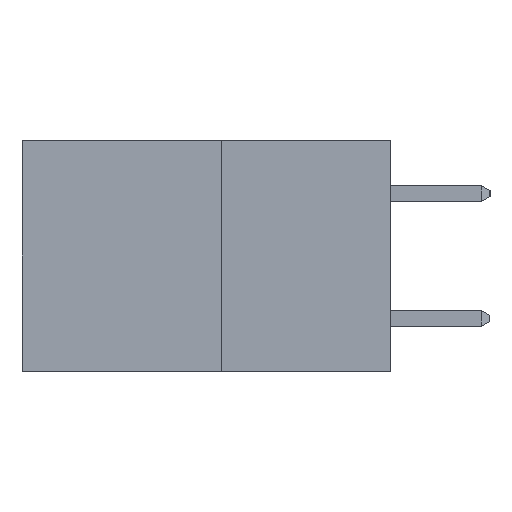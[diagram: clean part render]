
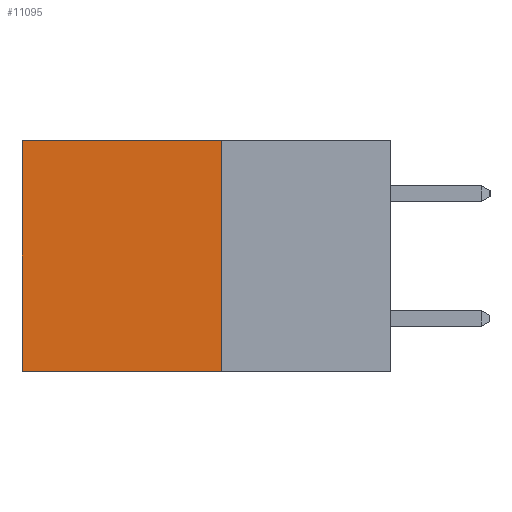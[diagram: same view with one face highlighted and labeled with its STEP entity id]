
A CAD part, left-side view. The second image highlights one B-rep face of the part: STEP entity #11095.
In plain terms, the highlighted planar face has unit normal (-1, 0, 0).
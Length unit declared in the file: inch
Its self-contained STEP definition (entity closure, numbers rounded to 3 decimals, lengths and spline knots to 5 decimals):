
#29 = LINE ( 'NONE', #15586, #6264 ) ;
#451 = ORIENTED_EDGE ( 'NONE', *, *, #4516, .T. ) ;
#937 = CARTESIAN_POINT ( 'NONE',  ( 0.277, 0.59, 0. ) ) ;
#2803 = EDGE_CURVE ( 'NONE', #3641, #4200, #3269, .T. ) ;
#3064 = DIRECTION ( 'NONE',  ( 1., 0., 0. ) ) ;
#3269 = LINE ( 'NONE', #3880, #9485 ) ;
#3363 = ORIENTED_EDGE ( 'NONE', *, *, #2803, .F. ) ;
#3641 = VERTEX_POINT ( 'NONE', #14148 ) ;
#3850 = VERTEX_POINT ( 'NONE', #6084 ) ;
#3880 = CARTESIAN_POINT ( 'NONE',  ( 0.277, 0.27, -0.37 ) ) ;
#4200 = VERTEX_POINT ( 'NONE', #7106 ) ;
#4208 = FACE_OUTER_BOUND ( 'NONE', #8446, .T. ) ;
#4516 = EDGE_CURVE ( 'NONE', #3641, #12582, #9625, .T. ) ;
#5011 = EDGE_CURVE ( 'NONE', #4200, #3850, #8862, .T. ) ;
#5184 = VECTOR ( 'NONE', #14505, 39.37008 ) ;
#5281 = DIRECTION ( 'NONE',  ( 0., 0., -1. ) ) ;
#5482 = AXIS2_PLACEMENT_3D ( 'NONE', #10503, #3064, #11690 ) ;
#5937 = ORIENTED_EDGE ( 'NONE', *, *, #7712, .T. ) ;
#6084 = CARTESIAN_POINT ( 'NONE',  ( 0.277, 0.59, -0.37 ) ) ;
#6264 = VECTOR ( 'NONE', #15557, 39.37008 ) ;
#7106 = CARTESIAN_POINT ( 'NONE',  ( 0.277, 0.27, -0.37 ) ) ;
#7712 = EDGE_CURVE ( 'NONE', #12582, #3850, #29, .T. ) ;
#8039 = PLANE ( 'NONE',  #5482 ) ;
#8446 = EDGE_LOOP ( 'NONE', ( #5937, #15397, #3363, #451 ) ) ;
#8862 = LINE ( 'NONE', #14587, #5184 ) ;
#9485 = VECTOR ( 'NONE', #5281, 39.37008 ) ;
#9625 = LINE ( 'NONE', #11759, #12398 ) ;
#10503 = CARTESIAN_POINT ( 'NONE',  ( 0.277, 0.27, -0.37 ) ) ;
#11095 = ADVANCED_FACE ( 'NONE', ( #4208 ), #8039, .F. ) ;
#11690 = DIRECTION ( 'NONE',  ( 0., 0., -1. ) ) ;
#11759 = CARTESIAN_POINT ( 'NONE',  ( 0.277, 0.27, 0. ) ) ;
#11859 = DIRECTION ( 'NONE',  ( 0., 1., 0. ) ) ;
#12398 = VECTOR ( 'NONE', #11859, 39.37008 ) ;
#12582 = VERTEX_POINT ( 'NONE', #937 ) ;
#14148 = CARTESIAN_POINT ( 'NONE',  ( 0.277, 0.27, 0. ) ) ;
#14505 = DIRECTION ( 'NONE',  ( 0., 1., 0. ) ) ;
#14587 = CARTESIAN_POINT ( 'NONE',  ( 0.277, 0.27, -0.37 ) ) ;
#15397 = ORIENTED_EDGE ( 'NONE', *, *, #5011, .F. ) ;
#15557 = DIRECTION ( 'NONE',  ( 0., 0., -1. ) ) ;
#15586 = CARTESIAN_POINT ( 'NONE',  ( 0.277, 0.59, -0.37 ) ) ;
